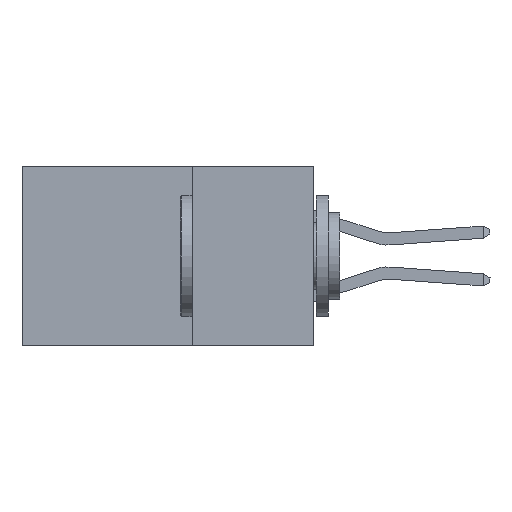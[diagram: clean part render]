
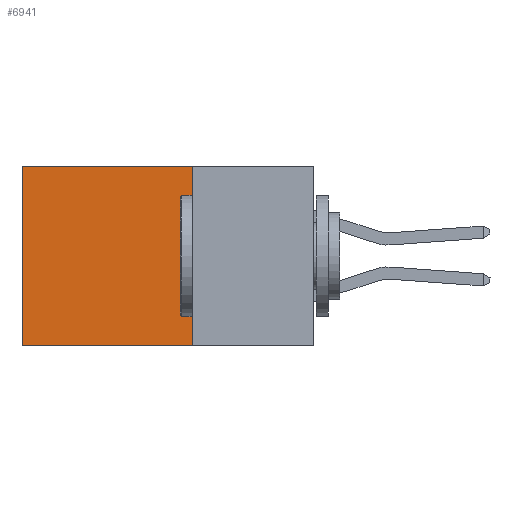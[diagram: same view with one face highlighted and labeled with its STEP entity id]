
A CAD part, left-side view. The second image highlights one B-rep face of the part: STEP entity #6941.
In plain terms, the highlighted planar face has unit normal (-1, 0, 0).
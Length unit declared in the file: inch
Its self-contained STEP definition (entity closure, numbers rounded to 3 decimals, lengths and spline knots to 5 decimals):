
#45 = CARTESIAN_POINT ( 'NONE',  ( 0.2875, 0.25, 0. ) ) ;
#610 = LINE ( 'NONE', #16204, #15129 ) ;
#1077 = ORIENTED_EDGE ( 'NONE', *, *, #8738, .T. ) ;
#1419 = FACE_OUTER_BOUND ( 'NONE', #23527, .T. ) ;
#1482 = DIRECTION ( 'NONE',  ( 0., 0., -1. ) ) ;
#2794 = CARTESIAN_POINT ( 'NONE',  ( 0.2875, 0.25, 0. ) ) ;
#4926 = VECTOR ( 'NONE', #23518, 39.37008 ) ;
#6302 = PLANE ( 'NONE',  #9056 ) ;
#6941 = ADVANCED_FACE ( 'NONE', ( #1419 ), #6302, .F. ) ;
#7873 = EDGE_CURVE ( 'NONE', #13481, #18073, #20111, .T. ) ;
#8415 = LINE ( 'NONE', #16261, #26790 ) ;
#8738 = EDGE_CURVE ( 'NONE', #13199, #10658, #20717, .T. ) ;
#9056 = AXIS2_PLACEMENT_3D ( 'NONE', #45, #23173, #14785 ) ;
#10658 = VERTEX_POINT ( 'NONE', #13795 ) ;
#13199 = VERTEX_POINT ( 'NONE', #26078 ) ;
#13382 = EDGE_CURVE ( 'NONE', #13199, #13481, #610, .T. ) ;
#13481 = VERTEX_POINT ( 'NONE', #20957 ) ;
#13795 = CARTESIAN_POINT ( 'NONE',  ( 0.2875, 0.6, 0. ) ) ;
#14235 = CARTESIAN_POINT ( 'NONE',  ( 0.2875, 0.25, -0.37 ) ) ;
#14785 = DIRECTION ( 'NONE',  ( 0., 0., -1. ) ) ;
#15129 = VECTOR ( 'NONE', #1482, 39.37008 ) ;
#15136 = CARTESIAN_POINT ( 'NONE',  ( 0.2875, 0.6, -0.37 ) ) ;
#16204 = CARTESIAN_POINT ( 'NONE',  ( 0.2875, 0.25, 0. ) ) ;
#16261 = CARTESIAN_POINT ( 'NONE',  ( 0.2875, 0.6, 0. ) ) ;
#17524 = ORIENTED_EDGE ( 'NONE', *, *, #21803, .T. ) ;
#18073 = VERTEX_POINT ( 'NONE', #15136 ) ;
#18246 = DIRECTION ( 'NONE',  ( 0., 0., -1. ) ) ;
#20111 = LINE ( 'NONE', #14235, #23375 ) ;
#20717 = LINE ( 'NONE', #2794, #4926 ) ;
#20957 = CARTESIAN_POINT ( 'NONE',  ( 0.2875, 0.25, -0.37 ) ) ;
#21267 = ORIENTED_EDGE ( 'NONE', *, *, #13382, .F. ) ;
#21803 = EDGE_CURVE ( 'NONE', #10658, #18073, #8415, .T. ) ;
#23173 = DIRECTION ( 'NONE',  ( 1., 0., 0. ) ) ;
#23375 = VECTOR ( 'NONE', #26512, 39.37008 ) ;
#23518 = DIRECTION ( 'NONE',  ( 0., 1., 0. ) ) ;
#23527 = EDGE_LOOP ( 'NONE', ( #17524, #25530, #21267, #1077 ) ) ;
#25530 = ORIENTED_EDGE ( 'NONE', *, *, #7873, .F. ) ;
#26078 = CARTESIAN_POINT ( 'NONE',  ( 0.2875, 0.25, 0. ) ) ;
#26512 = DIRECTION ( 'NONE',  ( 0., 1., 0. ) ) ;
#26790 = VECTOR ( 'NONE', #18246, 39.37008 ) ;
